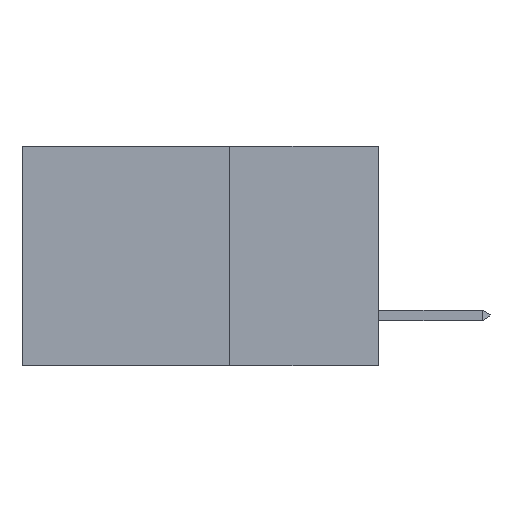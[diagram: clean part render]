
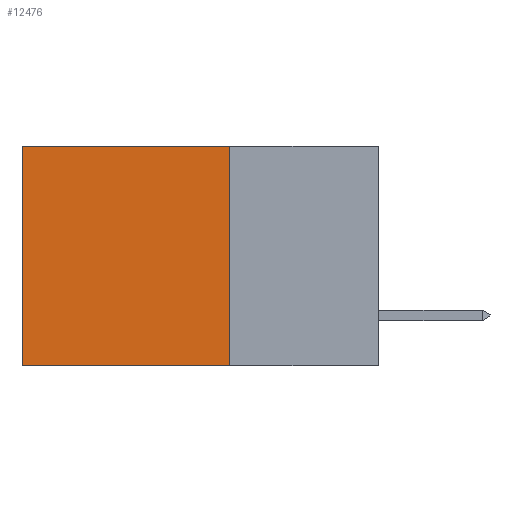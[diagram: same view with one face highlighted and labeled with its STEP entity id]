
A CAD part, left-side view. The second image highlights one B-rep face of the part: STEP entity #12476.
In plain terms, the highlighted planar face has unit normal (-1, 0, 0).
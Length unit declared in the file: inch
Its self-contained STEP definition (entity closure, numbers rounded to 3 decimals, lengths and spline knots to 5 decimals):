
#1153 = CARTESIAN_POINT ( 'NONE',  ( 0.298, 0.6, -0.37 ) ) ;
#1160 = EDGE_LOOP ( 'NONE', ( #6349, #20508, #10106, #19210 ) ) ;
#1329 = CARTESIAN_POINT ( 'NONE',  ( 0.298, 0.25, -0.37 ) ) ;
#1330 = EDGE_CURVE ( 'NONE', #10499, #9059, #12249, .T. ) ;
#2661 = DIRECTION ( 'NONE',  ( 0., 1., 0. ) ) ;
#2989 = CARTESIAN_POINT ( 'NONE',  ( 0.298, 0.6, 0. ) ) ;
#3485 = FACE_OUTER_BOUND ( 'NONE', #1160, .T. ) ;
#3697 = CARTESIAN_POINT ( 'NONE',  ( 0.298, 0.25, -0.37 ) ) ;
#4952 = CARTESIAN_POINT ( 'NONE',  ( 0.298, 0.6, 0. ) ) ;
#5353 = DIRECTION ( 'NONE',  ( 0., 0., -1. ) ) ;
#5686 = LINE ( 'NONE', #1329, #9569 ) ;
#5785 = DIRECTION ( 'NONE',  ( 1., 0., 0. ) ) ;
#6158 = EDGE_CURVE ( 'NONE', #16544, #19989, #7584, .T. ) ;
#6349 = ORIENTED_EDGE ( 'NONE', *, *, #1330, .T. ) ;
#6566 = VECTOR ( 'NONE', #5353, 39.37008 ) ;
#6693 = AXIS2_PLACEMENT_3D ( 'NONE', #15879, #5785, #11096 ) ;
#7584 = LINE ( 'NONE', #10087, #6566 ) ;
#7806 = VECTOR ( 'NONE', #21456, 39.37008 ) ;
#9059 = VERTEX_POINT ( 'NONE', #1153 ) ;
#9569 = VECTOR ( 'NONE', #10981, 39.37008 ) ;
#9771 = EDGE_CURVE ( 'NONE', #19989, #9059, #5686, .T. ) ;
#10087 = CARTESIAN_POINT ( 'NONE',  ( 0.298, 0.25, 0. ) ) ;
#10106 = ORIENTED_EDGE ( 'NONE', *, *, #6158, .F. ) ;
#10499 = VERTEX_POINT ( 'NONE', #2989 ) ;
#10981 = DIRECTION ( 'NONE',  ( 0., 1., 0. ) ) ;
#11096 = DIRECTION ( 'NONE',  ( 0., 0., -1. ) ) ;
#12249 = LINE ( 'NONE', #4952, #7806 ) ;
#12476 = ADVANCED_FACE ( 'NONE', ( #3485 ), #17310, .F. ) ;
#13643 = VECTOR ( 'NONE', #2661, 39.37008 ) ;
#14206 = CARTESIAN_POINT ( 'NONE',  ( 0.298, 0.25, 0. ) ) ;
#15879 = CARTESIAN_POINT ( 'NONE',  ( 0.298, 0.25, 0. ) ) ;
#15964 = LINE ( 'NONE', #14206, #13643 ) ;
#16544 = VERTEX_POINT ( 'NONE', #18044 ) ;
#17310 = PLANE ( 'NONE',  #6693 ) ;
#18044 = CARTESIAN_POINT ( 'NONE',  ( 0.298, 0.25, 0. ) ) ;
#19210 = ORIENTED_EDGE ( 'NONE', *, *, #20245, .T. ) ;
#19989 = VERTEX_POINT ( 'NONE', #3697 ) ;
#20245 = EDGE_CURVE ( 'NONE', #16544, #10499, #15964, .T. ) ;
#20508 = ORIENTED_EDGE ( 'NONE', *, *, #9771, .F. ) ;
#21456 = DIRECTION ( 'NONE',  ( 0., 0., -1. ) ) ;
